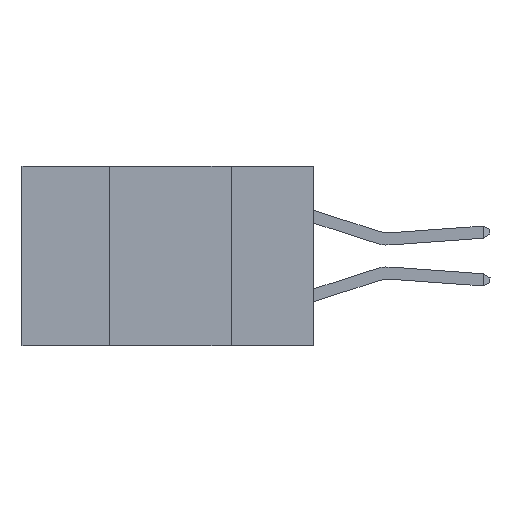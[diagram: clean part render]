
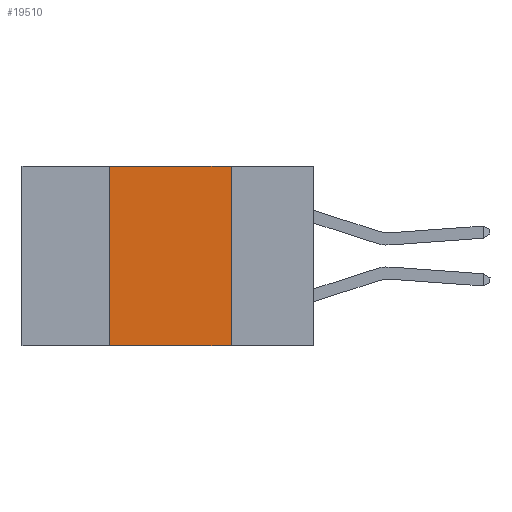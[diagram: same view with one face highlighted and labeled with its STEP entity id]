
A CAD part, left-side view. The second image highlights one B-rep face of the part: STEP entity #19510.
In plain terms, the highlighted planar face has unit normal (-1, 0, 0).
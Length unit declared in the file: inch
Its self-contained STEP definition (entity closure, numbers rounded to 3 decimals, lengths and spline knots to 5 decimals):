
#243 = DIRECTION ( 'NONE',  ( 0., -1., 0. ) ) ;
#1129 = VECTOR ( 'NONE', #33844, 39.37008 ) ;
#2059 = LINE ( 'NONE', #30940, #1129 ) ;
#2678 = EDGE_CURVE ( 'NONE', #11451, #18454, #2059, .T. ) ;
#2949 = EDGE_CURVE ( 'NONE', #16094, #11451, #30734, .T. ) ;
#2952 = EDGE_LOOP ( 'NONE', ( #31643, #32242, #17708, #11770 ) ) ;
#3687 = LINE ( 'NONE', #25119, #16436 ) ;
#4748 = PLANE ( 'NONE',  #17577 ) ;
#5314 = CARTESIAN_POINT ( 'NONE',  ( 0., 0.6, -0.37 ) ) ;
#6552 = LINE ( 'NONE', #5314, #13388 ) ;
#7684 = DIRECTION ( 'NONE',  ( 1., 0., 0. ) ) ;
#8948 = CARTESIAN_POINT ( 'NONE',  ( 0., 0.6, 0. ) ) ;
#11451 = VERTEX_POINT ( 'NONE', #21655 ) ;
#11770 = ORIENTED_EDGE ( 'NONE', *, *, #13915, .T. ) ;
#13388 = VECTOR ( 'NONE', #14108, 39.37008 ) ;
#13406 = FACE_OUTER_BOUND ( 'NONE', #2952, .T. ) ;
#13915 = EDGE_CURVE ( 'NONE', #25722, #18454, #6552, .T. ) ;
#14108 = DIRECTION ( 'NONE',  ( 0., -1., 0. ) ) ;
#16094 = VERTEX_POINT ( 'NONE', #21959 ) ;
#16436 = VECTOR ( 'NONE', #36547, 39.37008 ) ;
#17577 = AXIS2_PLACEMENT_3D ( 'NONE', #30836, #7684, #28016 ) ;
#17708 = ORIENTED_EDGE ( 'NONE', *, *, #32655, .F. ) ;
#18454 = VERTEX_POINT ( 'NONE', #20367 ) ;
#19510 = ADVANCED_FACE ( 'NONE', ( #13406 ), #4748, .F. ) ;
#20367 = CARTESIAN_POINT ( 'NONE',  ( 0., 0.17, -0.37 ) ) ;
#21655 = CARTESIAN_POINT ( 'NONE',  ( 0., 0.17, 0. ) ) ;
#21959 = CARTESIAN_POINT ( 'NONE',  ( 0., 0.42, 0. ) ) ;
#22067 = VECTOR ( 'NONE', #243, 39.37008 ) ;
#25119 = CARTESIAN_POINT ( 'NONE',  ( 0., 0.42, 0. ) ) ;
#25722 = VERTEX_POINT ( 'NONE', #27919 ) ;
#27919 = CARTESIAN_POINT ( 'NONE',  ( 0., 0.42, -0.37 ) ) ;
#28016 = DIRECTION ( 'NONE',  ( 0., 0., -1. ) ) ;
#30734 = LINE ( 'NONE', #8948, #22067 ) ;
#30836 = CARTESIAN_POINT ( 'NONE',  ( 0., 0.6, 0. ) ) ;
#30940 = CARTESIAN_POINT ( 'NONE',  ( 0., 0.17, 0. ) ) ;
#31643 = ORIENTED_EDGE ( 'NONE', *, *, #2678, .F. ) ;
#32242 = ORIENTED_EDGE ( 'NONE', *, *, #2949, .F. ) ;
#32655 = EDGE_CURVE ( 'NONE', #25722, #16094, #3687, .T. ) ;
#33844 = DIRECTION ( 'NONE',  ( 0., 0., -1. ) ) ;
#36547 = DIRECTION ( 'NONE',  ( 0., 0., 1. ) ) ;
